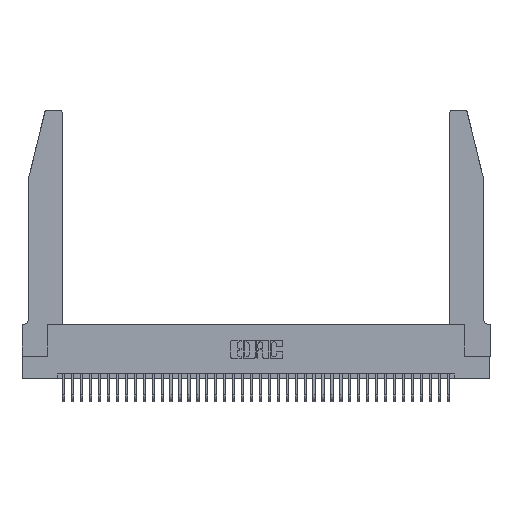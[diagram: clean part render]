
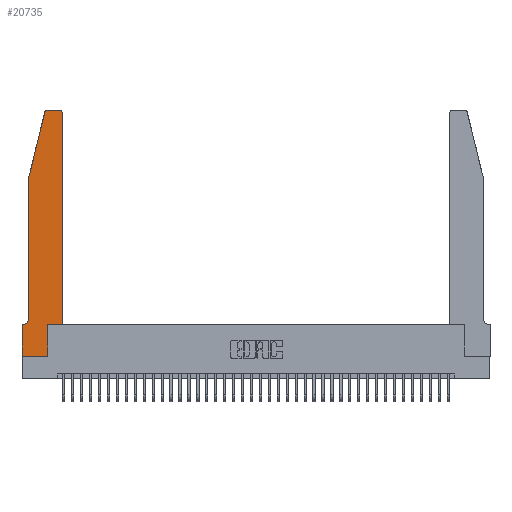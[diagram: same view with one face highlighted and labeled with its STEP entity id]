
A CAD part, top view. The second image highlights one B-rep face of the part: STEP entity #20735.
In plain terms, the highlighted planar face has unit normal (0, 0, 1).
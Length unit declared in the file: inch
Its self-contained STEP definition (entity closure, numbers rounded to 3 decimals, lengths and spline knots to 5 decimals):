
#333 = AXIS2_PLACEMENT_3D ( 'NONE', #26391, #8921, #29286 ) ;
#909 = EDGE_CURVE ( 'NONE', #27630, #22081, #23722, .T. ) ;
#1050 = CARTESIAN_POINT ( 'NONE',  ( 0.284, 2.75, 0.37 ) ) ;
#1217 = CARTESIAN_POINT ( 'NONE',  ( 0., 0.35, 0.37 ) ) ;
#1425 = CARTESIAN_POINT ( 'NONE',  ( 0.2865, 0., 0.37 ) ) ;
#1492 = ORIENTED_EDGE ( 'NONE', *, *, #6944, .T. ) ;
#1620 = CARTESIAN_POINT ( 'NONE',  ( 0.4505, 0.35, 0.37 ) ) ;
#2228 = CARTESIAN_POINT ( 'NONE',  ( 0.0055, 0.42, 0.37 ) ) ;
#3314 = ORIENTED_EDGE ( 'NONE', *, *, #8751, .T. ) ;
#3693 = DIRECTION ( 'NONE',  ( -1., 0., 0. ) ) ;
#3949 = VECTOR ( 'NONE', #4488, 39.37008 ) ;
#4146 = DIRECTION ( 'NONE',  ( 1., 0., 0. ) ) ;
#4160 = CARTESIAN_POINT ( 'NONE',  ( 0.4205, 2.72, 0.37 ) ) ;
#4184 = EDGE_LOOP ( 'NONE', ( #6476, #10211, #35305, #28039, #23004, #21628, #8917, #13682, #29667, #37415, #1492, #3314 ) ) ;
#4488 = DIRECTION ( 'NONE',  ( 0., -1., 0. ) ) ;
#4513 = EDGE_CURVE ( 'NONE', #5327, #27630, #32613, .T. ) ;
#4644 = CARTESIAN_POINT ( 'NONE',  ( 0.4505, 2.72, 0.37 ) ) ;
#5142 = DIRECTION ( 'NONE',  ( -1., 0., 0. ) ) ;
#5240 = CIRCLE ( 'NONE', #333, 0.03 ) ;
#5327 = VERTEX_POINT ( 'NONE', #7962 ) ;
#5702 = LINE ( 'NONE', #22288, #33952 ) ;
#6476 = ORIENTED_EDGE ( 'NONE', *, *, #17461, .T. ) ;
#6485 = FACE_OUTER_BOUND ( 'NONE', #4184, .T. ) ;
#6944 = EDGE_CURVE ( 'NONE', #14606, #29154, #22336, .T. ) ;
#7065 = DIRECTION ( 'NONE',  ( 1., 0., 0. ) ) ;
#7849 = VECTOR ( 'NONE', #10712, 39.37008 ) ;
#7962 = CARTESIAN_POINT ( 'NONE',  ( 0.0755, 2., 0.37 ) ) ;
#8121 = DIRECTION ( 'NONE',  ( 1., 0., 0. ) ) ;
#8751 = EDGE_CURVE ( 'NONE', #29154, #14350, #15330, .T. ) ;
#8917 = ORIENTED_EDGE ( 'NONE', *, *, #13654, .T. ) ;
#8921 = DIRECTION ( 'NONE',  ( 0., 0., 1. ) ) ;
#9336 = VECTOR ( 'NONE', #24539, 39.37008 ) ;
#10211 = ORIENTED_EDGE ( 'NONE', *, *, #28381, .T. ) ;
#10712 = DIRECTION ( 'NONE',  ( 1., 0., 0. ) ) ;
#11822 = VERTEX_POINT ( 'NONE', #1425 ) ;
#13269 = VECTOR ( 'NONE', #8121, 39.37008 ) ;
#13654 = EDGE_CURVE ( 'NONE', #14152, #26448, #34014, .T. ) ;
#13682 = ORIENTED_EDGE ( 'NONE', *, *, #20915, .T. ) ;
#14152 = VERTEX_POINT ( 'NONE', #21305 ) ;
#14350 = VERTEX_POINT ( 'NONE', #19387 ) ;
#14567 = VECTOR ( 'NONE', #33573, 39.37008 ) ;
#14606 = VERTEX_POINT ( 'NONE', #32172 ) ;
#15330 = CIRCLE ( 'NONE', #29604, 0.03 ) ;
#15531 = LINE ( 'NONE', #22300, #7849 ) ;
#15663 = PLANE ( 'NONE',  #37162 ) ;
#17461 = EDGE_CURVE ( 'NONE', #14350, #23114, #27734, .T. ) ;
#17984 = VECTOR ( 'NONE', #3693, 39.37008 ) ;
#19387 = CARTESIAN_POINT ( 'NONE',  ( 0.4205, 2.75, 0.37 ) ) ;
#19795 = VERTEX_POINT ( 'NONE', #20143 ) ;
#19834 = VERTEX_POINT ( 'NONE', #35065 ) ;
#20143 = CARTESIAN_POINT ( 'NONE',  ( 0.2865, 0.35, 0.37 ) ) ;
#20735 = ADVANCED_FACE ( 'NONE', ( #6485 ), #15663, .T. ) ;
#20915 = EDGE_CURVE ( 'NONE', #26448, #11822, #15531, .T. ) ;
#21305 = CARTESIAN_POINT ( 'NONE',  ( 0., 0.35, 0.37 ) ) ;
#21524 = DIRECTION ( 'NONE',  ( 0., 0., 1. ) ) ;
#21628 = ORIENTED_EDGE ( 'NONE', *, *, #34256, .T. ) ;
#21868 = CARTESIAN_POINT ( 'NONE',  ( 0., 0., 0.37 ) ) ;
#22081 = VERTEX_POINT ( 'NONE', #25433 ) ;
#22288 = CARTESIAN_POINT ( 'NONE',  ( 0.2865, 0.35, 0.37 ) ) ;
#22300 = CARTESIAN_POINT ( 'NONE',  ( 0., 0., 0.37 ) ) ;
#22336 = LINE ( 'NONE', #1620, #14567 ) ;
#22542 = DIRECTION ( 'NONE',  ( 0., 0., -1. ) ) ;
#23004 = ORIENTED_EDGE ( 'NONE', *, *, #909, .T. ) ;
#23114 = VERTEX_POINT ( 'NONE', #1050 ) ;
#23722 = CIRCLE ( 'NONE', #27349, 0.07 ) ;
#24019 = CARTESIAN_POINT ( 'NONE',  ( 0.0755, 0.35, 0.37 ) ) ;
#24083 = VECTOR ( 'NONE', #24969, 39.37008 ) ;
#24475 = DIRECTION ( 'NONE',  ( 0., 0., 1. ) ) ;
#24539 = DIRECTION ( 'NONE',  ( 0., -1., 0. ) ) ;
#24969 = DIRECTION ( 'NONE',  ( -0.239, -0.971, 0. ) ) ;
#25433 = CARTESIAN_POINT ( 'NONE',  ( 0.0055, 0.35, 0.37 ) ) ;
#26391 = CARTESIAN_POINT ( 'NONE',  ( 0.284, 2.72, 0.37 ) ) ;
#26448 = VERTEX_POINT ( 'NONE', #28560 ) ;
#26723 = LINE ( 'NONE', #24019, #17984 ) ;
#27349 = AXIS2_PLACEMENT_3D ( 'NONE', #2228, #22542, #5142 ) ;
#27515 = CARTESIAN_POINT ( 'NONE',  ( 0.0755, 2., 0.37 ) ) ;
#27630 = VERTEX_POINT ( 'NONE', #31415 ) ;
#27734 = LINE ( 'NONE', #34137, #34552 ) ;
#28039 = ORIENTED_EDGE ( 'NONE', *, *, #4513, .T. ) ;
#28166 = EDGE_CURVE ( 'NONE', #11822, #19795, #5702, .T. ) ;
#28381 = EDGE_CURVE ( 'NONE', #23114, #19834, #5240, .T. ) ;
#28560 = CARTESIAN_POINT ( 'NONE',  ( 0., 0., 0.37 ) ) ;
#29154 = VERTEX_POINT ( 'NONE', #4644 ) ;
#29286 = DIRECTION ( 'NONE',  ( 1., 0., 0. ) ) ;
#29604 = AXIS2_PLACEMENT_3D ( 'NONE', #4160, #24475, #7065 ) ;
#29667 = ORIENTED_EDGE ( 'NONE', *, *, #28166, .T. ) ;
#29850 = EDGE_CURVE ( 'NONE', #19795, #14606, #37421, .T. ) ;
#31115 = DIRECTION ( 'NONE',  ( 0., 1., 0. ) ) ;
#31415 = CARTESIAN_POINT ( 'NONE',  ( 0.0755, 0.42, 0.37 ) ) ;
#31443 = CARTESIAN_POINT ( 'NONE',  ( 0.4505, 0.35, 0.37 ) ) ;
#31889 = LINE ( 'NONE', #36415, #24083 ) ;
#32172 = CARTESIAN_POINT ( 'NONE',  ( 0.4505, 0.35, 0.37 ) ) ;
#32613 = LINE ( 'NONE', #27515, #9336 ) ;
#33573 = DIRECTION ( 'NONE',  ( 0., 1., 0. ) ) ;
#33952 = VECTOR ( 'NONE', #31115, 39.37008 ) ;
#34014 = LINE ( 'NONE', #21868, #3949 ) ;
#34137 = CARTESIAN_POINT ( 'NONE',  ( 0.2605, 2.75, 0.37 ) ) ;
#34256 = EDGE_CURVE ( 'NONE', #22081, #14152, #26723, .T. ) ;
#34552 = VECTOR ( 'NONE', #37035, 39.37008 ) ;
#35065 = CARTESIAN_POINT ( 'NONE',  ( 0.25487, 2.72718, 0.37 ) ) ;
#35305 = ORIENTED_EDGE ( 'NONE', *, *, #36217, .T. ) ;
#36217 = EDGE_CURVE ( 'NONE', #19834, #5327, #31889, .T. ) ;
#36415 = CARTESIAN_POINT ( 'NONE',  ( 0.0755, 2., 0.37 ) ) ;
#37035 = DIRECTION ( 'NONE',  ( -1., 0., 0. ) ) ;
#37162 = AXIS2_PLACEMENT_3D ( 'NONE', #1217, #21524, #4146 ) ;
#37415 = ORIENTED_EDGE ( 'NONE', *, *, #29850, .T. ) ;
#37421 = LINE ( 'NONE', #31443, #13269 ) ;
